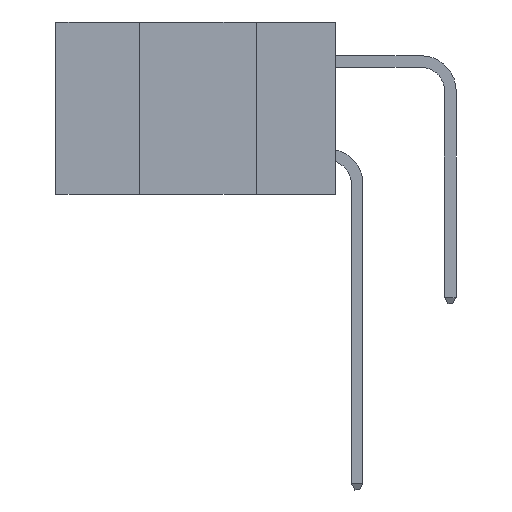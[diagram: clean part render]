
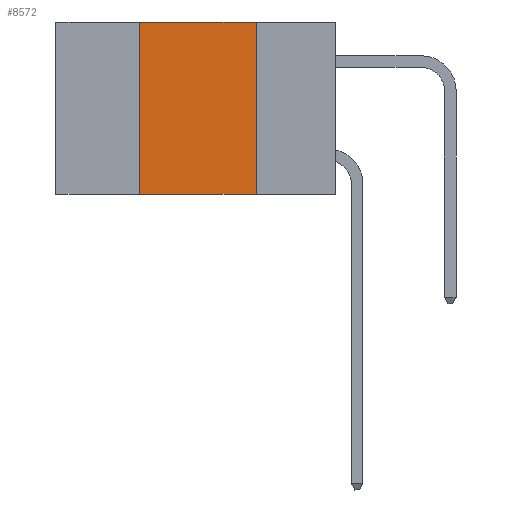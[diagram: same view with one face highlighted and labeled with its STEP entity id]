
A CAD part, left-side view. The second image highlights one B-rep face of the part: STEP entity #8572.
In plain terms, the highlighted planar face has unit normal (-1, 0, 0).
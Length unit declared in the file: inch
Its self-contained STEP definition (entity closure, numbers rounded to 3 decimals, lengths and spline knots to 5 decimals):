
#17 = DIRECTION ( 'NONE',  ( 1., 0., 0. ) ) ;
#265 = AXIS2_PLACEMENT_3D ( 'NONE', #9283, #17, #8166 ) ;
#980 = CARTESIAN_POINT ( 'NONE',  ( 0., 0.6, 0. ) ) ;
#1240 = LINE ( 'NONE', #980, #8925 ) ;
#1857 = CARTESIAN_POINT ( 'NONE',  ( 0., 0.17, -0.37 ) ) ;
#2137 = DIRECTION ( 'NONE',  ( 0., 0., -1. ) ) ;
#2249 = ORIENTED_EDGE ( 'NONE', *, *, #3450, .F. ) ;
#2261 = EDGE_CURVE ( 'NONE', #3106, #11027, #1240, .T. ) ;
#2644 = CARTESIAN_POINT ( 'NONE',  ( 0., 0.6, -0.37 ) ) ;
#3089 = EDGE_CURVE ( 'NONE', #10269, #5202, #6849, .T. ) ;
#3106 = VERTEX_POINT ( 'NONE', #6567 ) ;
#3450 = EDGE_CURVE ( 'NONE', #11027, #5202, #5845, .T. ) ;
#3680 = VECTOR ( 'NONE', #7441, 39.37008 ) ;
#4189 = CARTESIAN_POINT ( 'NONE',  ( 0., 0.17, 0. ) ) ;
#4616 = PLANE ( 'NONE',  #265 ) ;
#4938 = ORIENTED_EDGE ( 'NONE', *, *, #3089, .T. ) ;
#4940 = CARTESIAN_POINT ( 'NONE',  ( 0., 0.17, 0. ) ) ;
#5123 = VECTOR ( 'NONE', #2137, 39.37008 ) ;
#5202 = VERTEX_POINT ( 'NONE', #1857 ) ;
#5845 = LINE ( 'NONE', #4940, #5123 ) ;
#6324 = LINE ( 'NONE', #10645, #8946 ) ;
#6567 = CARTESIAN_POINT ( 'NONE',  ( 0., 0.42, 0. ) ) ;
#6849 = LINE ( 'NONE', #2644, #3680 ) ;
#6878 = DIRECTION ( 'NONE',  ( 0., 0., 1. ) ) ;
#7114 = EDGE_LOOP ( 'NONE', ( #2249, #9740, #11153, #4938 ) ) ;
#7441 = DIRECTION ( 'NONE',  ( 0., -1., 0. ) ) ;
#7533 = CARTESIAN_POINT ( 'NONE',  ( 0., 0.42, -0.37 ) ) ;
#8078 = FACE_OUTER_BOUND ( 'NONE', #7114, .T. ) ;
#8166 = DIRECTION ( 'NONE',  ( 0., 0., -1. ) ) ;
#8572 = ADVANCED_FACE ( 'NONE', ( #8078 ), #4616, .F. ) ;
#8925 = VECTOR ( 'NONE', #9266, 39.37008 ) ;
#8946 = VECTOR ( 'NONE', #6878, 39.37008 ) ;
#8976 = EDGE_CURVE ( 'NONE', #10269, #3106, #6324, .T. ) ;
#9266 = DIRECTION ( 'NONE',  ( 0., -1., 0. ) ) ;
#9283 = CARTESIAN_POINT ( 'NONE',  ( 0., 0.6, 0. ) ) ;
#9740 = ORIENTED_EDGE ( 'NONE', *, *, #2261, .F. ) ;
#10269 = VERTEX_POINT ( 'NONE', #7533 ) ;
#10645 = CARTESIAN_POINT ( 'NONE',  ( 0., 0.42, 0. ) ) ;
#11027 = VERTEX_POINT ( 'NONE', #4189 ) ;
#11153 = ORIENTED_EDGE ( 'NONE', *, *, #8976, .F. ) ;
